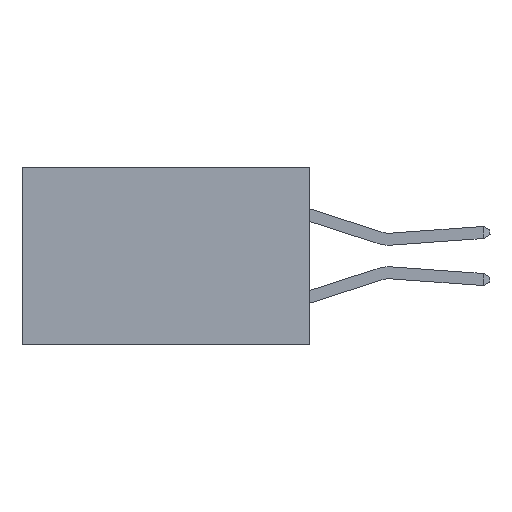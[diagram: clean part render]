
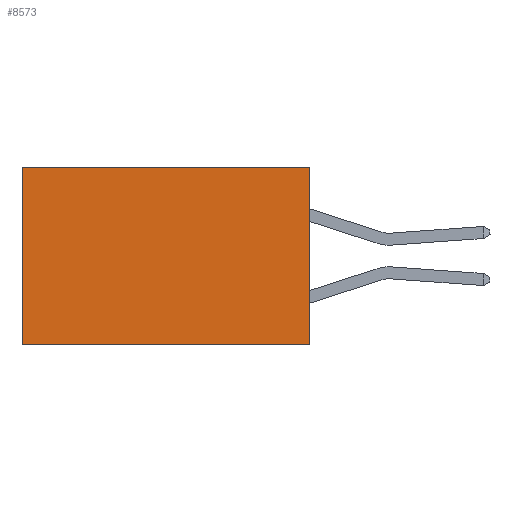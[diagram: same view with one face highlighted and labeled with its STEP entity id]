
A CAD part, left-side view. The second image highlights one B-rep face of the part: STEP entity #8573.
In plain terms, the highlighted planar face has unit normal (-1, 0, 0).
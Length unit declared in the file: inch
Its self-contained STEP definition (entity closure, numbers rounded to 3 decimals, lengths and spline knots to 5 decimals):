
#841 = VECTOR ( 'NONE', #3688, 39.37008 ) ;
#1083 = DIRECTION ( 'NONE',  ( 0., 1., 0. ) ) ;
#1189 = VERTEX_POINT ( 'NONE', #2532 ) ;
#1244 = CARTESIAN_POINT ( 'NONE',  ( 0.2615, 0.6, 0. ) ) ;
#1815 = CARTESIAN_POINT ( 'NONE',  ( 0.2615, 0., -0.37 ) ) ;
#1972 = LINE ( 'NONE', #1815, #7043 ) ;
#1992 = CARTESIAN_POINT ( 'NONE',  ( 0.2615, 0., -0.37 ) ) ;
#2028 = VERTEX_POINT ( 'NONE', #1244 ) ;
#2326 = ORIENTED_EDGE ( 'NONE', *, *, #10400, .F. ) ;
#2502 = DIRECTION ( 'NONE',  ( 0., 0., -1. ) ) ;
#2532 = CARTESIAN_POINT ( 'NONE',  ( 0.2615, 0., 0. ) ) ;
#2663 = ORIENTED_EDGE ( 'NONE', *, *, #5358, .T. ) ;
#3342 = EDGE_CURVE ( 'NONE', #1189, #7327, #10051, .T. ) ;
#3454 = VERTEX_POINT ( 'NONE', #10324 ) ;
#3688 = DIRECTION ( 'NONE',  ( 0., 0., -1. ) ) ;
#4518 = EDGE_LOOP ( 'NONE', ( #8162, #2326, #6552, #2663 ) ) ;
#4585 = CARTESIAN_POINT ( 'NONE',  ( 0.2615, 0.6, -0.37 ) ) ;
#5358 = EDGE_CURVE ( 'NONE', #1189, #2028, #7312, .T. ) ;
#6019 = CARTESIAN_POINT ( 'NONE',  ( 0.2615, 0., -0.37 ) ) ;
#6183 = AXIS2_PLACEMENT_3D ( 'NONE', #8713, #8107, #2502 ) ;
#6242 = CARTESIAN_POINT ( 'NONE',  ( 0.2615, 0., 0. ) ) ;
#6449 = VECTOR ( 'NONE', #9653, 39.37008 ) ;
#6552 = ORIENTED_EDGE ( 'NONE', *, *, #3342, .F. ) ;
#6699 = DIRECTION ( 'NONE',  ( 0., 0., -1. ) ) ;
#7043 = VECTOR ( 'NONE', #1083, 39.37008 ) ;
#7312 = LINE ( 'NONE', #6242, #6449 ) ;
#7327 = VERTEX_POINT ( 'NONE', #1992 ) ;
#7787 = LINE ( 'NONE', #4585, #841 ) ;
#8107 = DIRECTION ( 'NONE',  ( 1., 0., 0. ) ) ;
#8129 = VECTOR ( 'NONE', #6699, 39.37008 ) ;
#8162 = ORIENTED_EDGE ( 'NONE', *, *, #9323, .T. ) ;
#8573 = ADVANCED_FACE ( 'NONE', ( #9711 ), #8762, .F. ) ;
#8713 = CARTESIAN_POINT ( 'NONE',  ( 0.2615, 0., -0.37 ) ) ;
#8762 = PLANE ( 'NONE',  #6183 ) ;
#9323 = EDGE_CURVE ( 'NONE', #2028, #3454, #7787, .T. ) ;
#9653 = DIRECTION ( 'NONE',  ( 0., 1., 0. ) ) ;
#9711 = FACE_OUTER_BOUND ( 'NONE', #4518, .T. ) ;
#10051 = LINE ( 'NONE', #6019, #8129 ) ;
#10324 = CARTESIAN_POINT ( 'NONE',  ( 0.2615, 0.6, -0.37 ) ) ;
#10400 = EDGE_CURVE ( 'NONE', #7327, #3454, #1972, .T. ) ;
